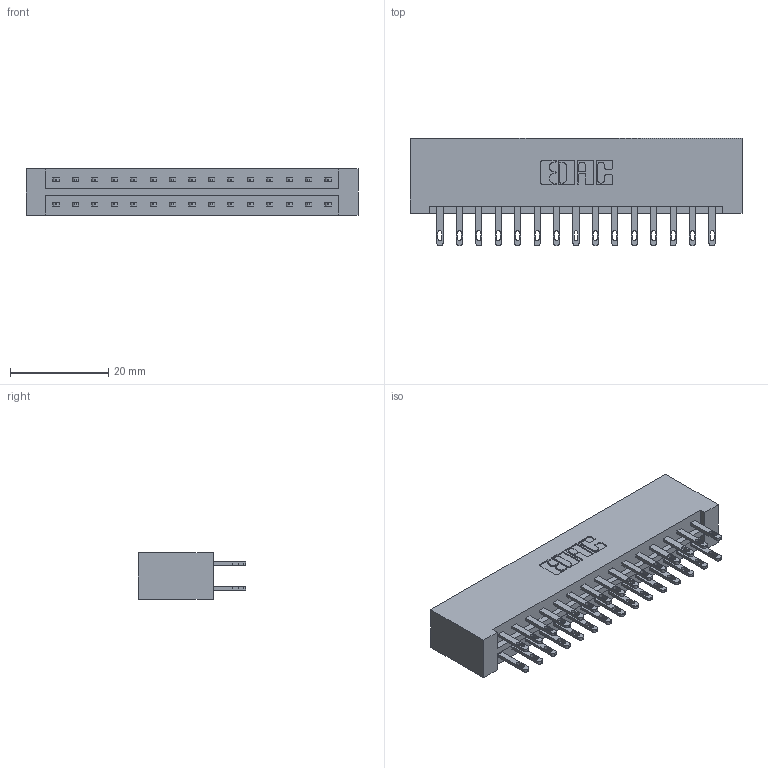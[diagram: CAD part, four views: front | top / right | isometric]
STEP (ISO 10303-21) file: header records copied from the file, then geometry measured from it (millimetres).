
FILE_DESCRIPTION (( 'STEP AP203' ), '1' );
FILE_NAME ('333-030-500-201.STEP', '2018-08-02T16:56:56', ( '' ), ( '' ), 'SwSTEP 2.0', 'SolidWorks 2016', '' );
FILE_SCHEMA (( 'CONFIG_CONTROL_DESIGN' ));
Length unit declared in the file: inch
Products named in the file (3): 345-292-001_345-293-100; 333-030-500-201; 333 Part_Lugless
Assembly tree (31 placements, depth 2):
  333-030-500-201
    333 Part_Lugless
    345-292-001_345-293-100  x30
Bounding box: 67.69 x 21.85 x 9.4 mm (x, y, z)
Volume: 7382.3 mm3; surface area: 8792 mm2
Topology: 31 solids, 31 shells, 1546 faces, 4697 edges, 3130 vertices
Faces by surface type: plane 966, cylinder 580
Entity records: 12795 total; most frequent: CARTESIAN_POINT 2150, ORIENTED_EDGE 2086, DIRECTION 1879, EDGE_CURVE 1043, VECTOR 919, LINE 919, VERTEX_POINT 694, AXIS2_PLACEMENT_3D 480
